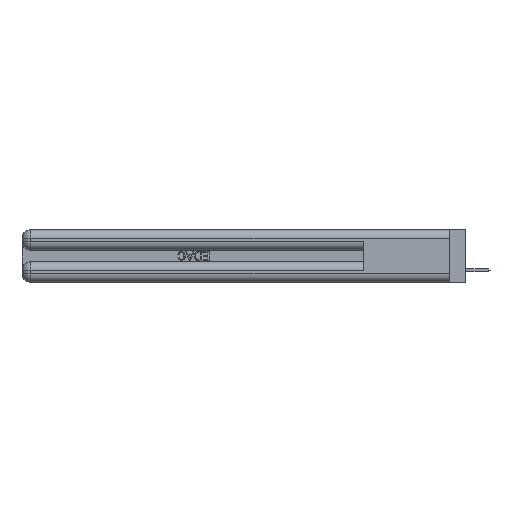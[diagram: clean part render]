
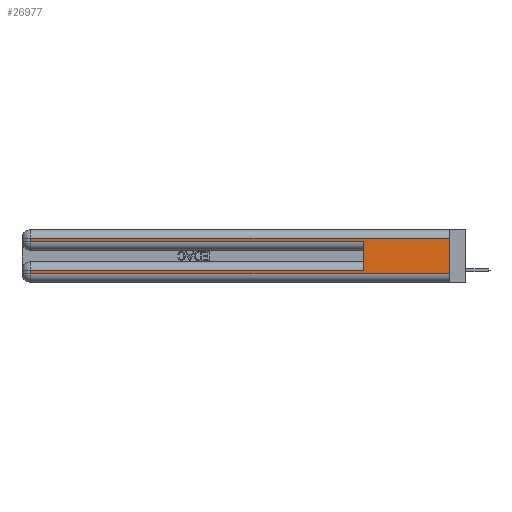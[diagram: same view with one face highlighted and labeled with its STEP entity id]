
A CAD part, left-side view. The second image highlights one B-rep face of the part: STEP entity #26977.
In plain terms, the highlighted planar face has unit normal (-1, 0, 0).
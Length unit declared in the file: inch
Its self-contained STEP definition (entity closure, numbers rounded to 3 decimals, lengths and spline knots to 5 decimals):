
#88 = EDGE_CURVE ( 'NONE', #33045, #14129, #37041, .T. ) ;
#432 = VECTOR ( 'NONE', #3663, 39.37008 ) ;
#1122 = EDGE_CURVE ( 'NONE', #14129, #36550, #18432, .T. ) ;
#2351 = CARTESIAN_POINT ( 'NONE',  ( 0., 0.6, 0.085 ) ) ;
#2768 = PLANE ( 'NONE',  #22307 ) ;
#2911 = ORIENTED_EDGE ( 'NONE', *, *, #35085, .F. ) ;
#3362 = VECTOR ( 'NONE', #7200, 39.37008 ) ;
#3368 = CARTESIAN_POINT ( 'NONE',  ( 0., 0., 0.31 ) ) ;
#3663 = DIRECTION ( 'NONE',  ( 0., 0., -1. ) ) ;
#3712 = VERTEX_POINT ( 'NONE', #28916 ) ;
#4281 = ORIENTED_EDGE ( 'NONE', *, *, #13408, .T. ) ;
#4300 = LINE ( 'NONE', #16270, #3362 ) ;
#5324 = DIRECTION ( 'NONE',  ( 1., 0., 0. ) ) ;
#6139 = CARTESIAN_POINT ( 'NONE',  ( 0., 0.6, 0.145 ) ) ;
#6217 = CARTESIAN_POINT ( 'NONE',  ( 0., 2.94, 0.37 ) ) ;
#7162 = VERTEX_POINT ( 'NONE', #11230 ) ;
#7200 = DIRECTION ( 'NONE',  ( 0., 1., 0. ) ) ;
#7218 = VERTEX_POINT ( 'NONE', #8737 ) ;
#7424 = VERTEX_POINT ( 'NONE', #2351 ) ;
#7797 = LINE ( 'NONE', #14632, #36459 ) ;
#8139 = DIRECTION ( 'NONE',  ( 0., -1., 0. ) ) ;
#8294 = CARTESIAN_POINT ( 'NONE',  ( 0., 0., 0.085 ) ) ;
#8394 = CARTESIAN_POINT ( 'NONE',  ( 0., 2.94, 0.285 ) ) ;
#8638 = EDGE_LOOP ( 'NONE', ( #2911, #16736, #23962, #12170, #22524, #4281, #14855, #16654 ) ) ;
#8737 = CARTESIAN_POINT ( 'NONE',  ( 0., 2.94, 0.085 ) ) ;
#9415 = DIRECTION ( 'NONE',  ( 0., 0., 1. ) ) ;
#11230 = CARTESIAN_POINT ( 'NONE',  ( 0., 0., 0.06 ) ) ;
#11366 = CARTESIAN_POINT ( 'NONE',  ( 0., 0., 0.06 ) ) ;
#11427 = VECTOR ( 'NONE', #9415, 39.37008 ) ;
#11643 = DIRECTION ( 'NONE',  ( 0., 1., 0. ) ) ;
#12165 = DIRECTION ( 'NONE',  ( 0., -1., 0. ) ) ;
#12170 = ORIENTED_EDGE ( 'NONE', *, *, #1122, .T. ) ;
#13408 = EDGE_CURVE ( 'NONE', #7424, #7218, #31848, .T. ) ;
#14129 = VERTEX_POINT ( 'NONE', #8394 ) ;
#14238 = LINE ( 'NONE', #6139, #11427 ) ;
#14632 = CARTESIAN_POINT ( 'NONE',  ( 0., 2.94, 0.37 ) ) ;
#14855 = ORIENTED_EDGE ( 'NONE', *, *, #31704, .T. ) ;
#16270 = CARTESIAN_POINT ( 'NONE',  ( 0., 0., 0.31 ) ) ;
#16654 = ORIENTED_EDGE ( 'NONE', *, *, #28087, .T. ) ;
#16736 = ORIENTED_EDGE ( 'NONE', *, *, #35464, .T. ) ;
#17701 = VERTEX_POINT ( 'NONE', #3368 ) ;
#18227 = LINE ( 'NONE', #32042, #36231 ) ;
#18432 = LINE ( 'NONE', #26858, #29472 ) ;
#20472 = DIRECTION ( 'NONE',  ( 0., 0., -1. ) ) ;
#22307 = AXIS2_PLACEMENT_3D ( 'NONE', #35320, #5324, #32087 ) ;
#22524 = ORIENTED_EDGE ( 'NONE', *, *, #30017, .F. ) ;
#23633 = FACE_OUTER_BOUND ( 'NONE', #8638, .T. ) ;
#23962 = ORIENTED_EDGE ( 'NONE', *, *, #88, .T. ) ;
#25265 = VECTOR ( 'NONE', #11643, 39.37008 ) ;
#25382 = CARTESIAN_POINT ( 'NONE',  ( 0., 2.94, 0.31 ) ) ;
#26858 = CARTESIAN_POINT ( 'NONE',  ( 0., 0., 0.285 ) ) ;
#26977 = ADVANCED_FACE ( 'NONE', ( #23633 ), #2768, .F. ) ;
#28087 = EDGE_CURVE ( 'NONE', #3712, #7162, #28650, .T. ) ;
#28170 = VECTOR ( 'NONE', #8139, 39.37008 ) ;
#28650 = LINE ( 'NONE', #11366, #28170 ) ;
#28916 = CARTESIAN_POINT ( 'NONE',  ( 0., 2.94, 0.06 ) ) ;
#29472 = VECTOR ( 'NONE', #12165, 39.37008 ) ;
#30017 = EDGE_CURVE ( 'NONE', #7424, #36550, #14238, .T. ) ;
#31704 = EDGE_CURVE ( 'NONE', #7218, #3712, #7797, .T. ) ;
#31848 = LINE ( 'NONE', #8294, #25265 ) ;
#32042 = CARTESIAN_POINT ( 'NONE',  ( 0., 0., 0.37 ) ) ;
#32087 = DIRECTION ( 'NONE',  ( 0., 0., -1. ) ) ;
#33045 = VERTEX_POINT ( 'NONE', #25382 ) ;
#35029 = DIRECTION ( 'NONE',  ( 0., 0., -1. ) ) ;
#35085 = EDGE_CURVE ( 'NONE', #17701, #7162, #18227, .T. ) ;
#35320 = CARTESIAN_POINT ( 'NONE',  ( 0., 0., 0.37 ) ) ;
#35464 = EDGE_CURVE ( 'NONE', #17701, #33045, #4300, .T. ) ;
#36231 = VECTOR ( 'NONE', #35029, 39.37008 ) ;
#36459 = VECTOR ( 'NONE', #20472, 39.37008 ) ;
#36550 = VERTEX_POINT ( 'NONE', #37125 ) ;
#37041 = LINE ( 'NONE', #6217, #432 ) ;
#37125 = CARTESIAN_POINT ( 'NONE',  ( 0., 0.6, 0.285 ) ) ;
